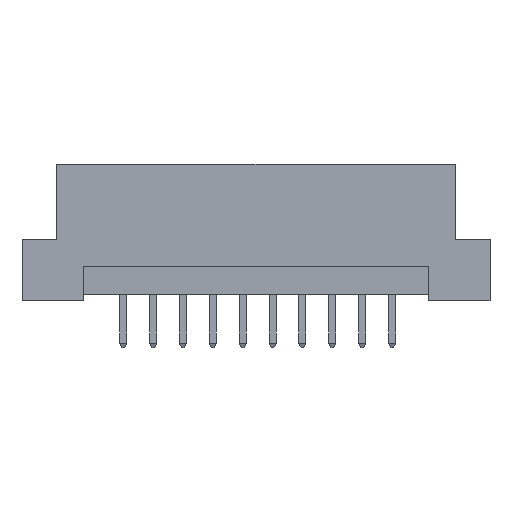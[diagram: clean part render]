
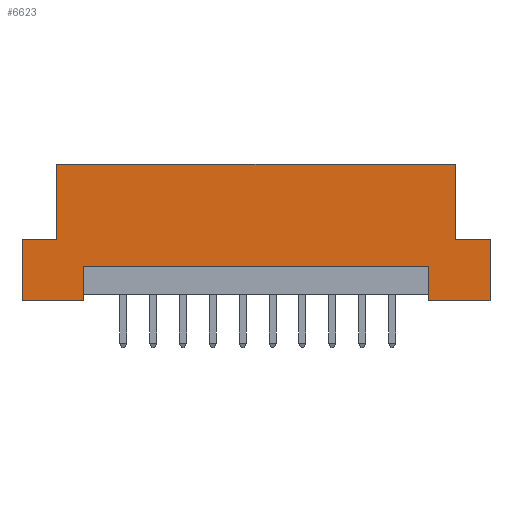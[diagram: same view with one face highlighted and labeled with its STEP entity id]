
A CAD part, front view. The second image highlights one B-rep face of the part: STEP entity #6623.
In plain terms, the highlighted planar face has unit normal (0, -1, 0).
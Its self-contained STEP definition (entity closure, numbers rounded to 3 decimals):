
#6 = EDGE_CURVE ( 'NONE', #1249, #6115, #4848, .T. ) ;
#70 = LINE ( 'NONE', #2786, #2813 ) ;
#89 = ORIENTED_EDGE ( 'NONE', *, *, #6, .F. ) ;
#136 = EDGE_CURVE ( 'NONE', #4569, #6546, #3872, .T. ) ;
#197 = CARTESIAN_POINT ( 'NONE',  ( 14.69, 0., 0. ) ) ;
#205 = EDGE_CURVE ( 'NONE', #6596, #249, #2194, .T. ) ;
#227 = LINE ( 'NONE', #7023, #6987 ) ;
#249 = VERTEX_POINT ( 'NONE', #197 ) ;
#285 = DIRECTION ( 'NONE',  ( 0., 0., 1. ) ) ;
#328 = PLANE ( 'NONE',  #820 ) ;
#412 = DIRECTION ( 'NONE',  ( 1., 0., 0. ) ) ;
#429 = CARTESIAN_POINT ( 'NONE',  ( 16.94, 0., 5.2 ) ) ;
#633 = LINE ( 'NONE', #2880, #651 ) ;
#637 = CARTESIAN_POINT ( 'NONE',  ( -19.9, 0., 0. ) ) ;
#649 = VERTEX_POINT ( 'NONE', #3262 ) ;
#651 = VECTOR ( 'NONE', #6717, 1000. ) ;
#717 = CARTESIAN_POINT ( 'NONE',  ( 16.94, 0., 5.2 ) ) ;
#820 = AXIS2_PLACEMENT_3D ( 'NONE', #3805, #5403, #285 ) ;
#832 = DIRECTION ( 'NONE',  ( 0., 0., 1. ) ) ;
#866 = CARTESIAN_POINT ( 'NONE',  ( -19.9, 0., 0. ) ) ;
#998 = VERTEX_POINT ( 'NONE', #6518 ) ;
#1003 = EDGE_CURVE ( 'NONE', #6596, #4569, #5958, .T. ) ;
#1139 = EDGE_CURVE ( 'NONE', #5702, #4006, #1870, .T. ) ;
#1249 = VERTEX_POINT ( 'NONE', #637 ) ;
#1346 = DIRECTION ( 'NONE',  ( 1., 0., 0. ) ) ;
#1409 = VECTOR ( 'NONE', #5511, 1000. ) ;
#1461 = VECTOR ( 'NONE', #832, 1000. ) ;
#1639 = ORIENTED_EDGE ( 'NONE', *, *, #205, .T. ) ;
#1870 = LINE ( 'NONE', #3524, #4926 ) ;
#2071 = VECTOR ( 'NONE', #5396, 1000. ) ;
#2151 = VERTEX_POINT ( 'NONE', #3751 ) ;
#2194 = LINE ( 'NONE', #6733, #7275 ) ;
#2226 = CARTESIAN_POINT ( 'NONE',  ( -14.69, 0., 0.5 ) ) ;
#2272 = VECTOR ( 'NONE', #3102, 1000. ) ;
#2786 = CARTESIAN_POINT ( 'NONE',  ( -16.94, 0., 5.2 ) ) ;
#2813 = VECTOR ( 'NONE', #6864, 1000. ) ;
#2865 = ORIENTED_EDGE ( 'NONE', *, *, #7058, .F. ) ;
#2880 = CARTESIAN_POINT ( 'NONE',  ( -19.9, 0., 0. ) ) ;
#2933 = ORIENTED_EDGE ( 'NONE', *, *, #136, .F. ) ;
#3102 = DIRECTION ( 'NONE',  ( -1., 0., 0. ) ) ;
#3109 = CARTESIAN_POINT ( 'NONE',  ( 14.69, 0., 2.9 ) ) ;
#3138 = EDGE_CURVE ( 'NONE', #4006, #249, #5955, .T. ) ;
#3166 = CARTESIAN_POINT ( 'NONE',  ( -19.9, 0., 11.6 ) ) ;
#3174 = VERTEX_POINT ( 'NONE', #717 ) ;
#3202 = VECTOR ( 'NONE', #412, 1000. ) ;
#3262 = CARTESIAN_POINT ( 'NONE',  ( -16.94, 0., 5.2 ) ) ;
#3363 = CARTESIAN_POINT ( 'NONE',  ( 19.9, 0., 0. ) ) ;
#3495 = ORIENTED_EDGE ( 'NONE', *, *, #4456, .F. ) ;
#3524 = CARTESIAN_POINT ( 'NONE',  ( 19.9, 0., 0. ) ) ;
#3733 = CARTESIAN_POINT ( 'NONE',  ( -14.69, 0., 2.9 ) ) ;
#3751 = CARTESIAN_POINT ( 'NONE',  ( 16.94, 0., 11.6 ) ) ;
#3805 = CARTESIAN_POINT ( 'NONE',  ( -19.9, 0., 11.6 ) ) ;
#3861 = LINE ( 'NONE', #3166, #3202 ) ;
#3872 = LINE ( 'NONE', #2226, #6681 ) ;
#4006 = VERTEX_POINT ( 'NONE', #3363 ) ;
#4076 = ORIENTED_EDGE ( 'NONE', *, *, #7041, .F. ) ;
#4236 = ORIENTED_EDGE ( 'NONE', *, *, #1003, .F. ) ;
#4257 = CARTESIAN_POINT ( 'NONE',  ( -19.9, 0., 5.2 ) ) ;
#4360 = FACE_OUTER_BOUND ( 'NONE', #5025, .T. ) ;
#4456 = EDGE_CURVE ( 'NONE', #6546, #1249, #633, .T. ) ;
#4569 = VERTEX_POINT ( 'NONE', #3733 ) ;
#4654 = DIRECTION ( 'NONE',  ( 0., 0., -1. ) ) ;
#4848 = LINE ( 'NONE', #7107, #1461 ) ;
#4870 = ORIENTED_EDGE ( 'NONE', *, *, #6548, .T. ) ;
#4926 = VECTOR ( 'NONE', #4654, 1000. ) ;
#5025 = EDGE_LOOP ( 'NONE', ( #4236, #1639, #5747, #6756, #2865, #4870, #5187, #6904, #4076, #89, #3495, #2933 ) ) ;
#5026 = DIRECTION ( 'NONE',  ( 0., 0., -1. ) ) ;
#5187 = ORIENTED_EDGE ( 'NONE', *, *, #7216, .F. ) ;
#5396 = DIRECTION ( 'NONE',  ( -1., 0., 0. ) ) ;
#5403 = DIRECTION ( 'NONE',  ( 0., 1., 0. ) ) ;
#5418 = CARTESIAN_POINT ( 'NONE',  ( 19.9, 0., 5.2 ) ) ;
#5511 = DIRECTION ( 'NONE',  ( 0., 0., 1. ) ) ;
#5558 = VECTOR ( 'NONE', #1346, 1000. ) ;
#5702 = VERTEX_POINT ( 'NONE', #5418 ) ;
#5747 = ORIENTED_EDGE ( 'NONE', *, *, #3138, .F. ) ;
#5955 = LINE ( 'NONE', #866, #2272 ) ;
#5958 = LINE ( 'NONE', #3109, #2071 ) ;
#6038 = LINE ( 'NONE', #429, #1409 ) ;
#6105 = DIRECTION ( 'NONE',  ( 0., 0., -1. ) ) ;
#6115 = VERTEX_POINT ( 'NONE', #4257 ) ;
#6269 = EDGE_CURVE ( 'NONE', #649, #998, #70, .T. ) ;
#6470 = DIRECTION ( 'NONE',  ( 1., 0., 0. ) ) ;
#6518 = CARTESIAN_POINT ( 'NONE',  ( -16.94, 0., 11.6 ) ) ;
#6546 = VERTEX_POINT ( 'NONE', #7115 ) ;
#6548 = EDGE_CURVE ( 'NONE', #3174, #2151, #6038, .T. ) ;
#6596 = VERTEX_POINT ( 'NONE', #7228 ) ;
#6623 = ADVANCED_FACE ( 'NONE', ( #4360 ), #328, .F. ) ;
#6681 = VECTOR ( 'NONE', #5026, 1000. ) ;
#6717 = DIRECTION ( 'NONE',  ( -1., 0., 0. ) ) ;
#6733 = CARTESIAN_POINT ( 'NONE',  ( 14.69, 0., 0.5 ) ) ;
#6756 = ORIENTED_EDGE ( 'NONE', *, *, #1139, .F. ) ;
#6864 = DIRECTION ( 'NONE',  ( 0., 0., 1. ) ) ;
#6904 = ORIENTED_EDGE ( 'NONE', *, *, #6269, .F. ) ;
#6987 = VECTOR ( 'NONE', #6470, 1000. ) ;
#6990 = CARTESIAN_POINT ( 'NONE',  ( -19.9, 0., 5.2 ) ) ;
#7023 = CARTESIAN_POINT ( 'NONE',  ( 19.9, 0., 5.2 ) ) ;
#7041 = EDGE_CURVE ( 'NONE', #6115, #649, #7135, .T. ) ;
#7058 = EDGE_CURVE ( 'NONE', #3174, #5702, #227, .T. ) ;
#7107 = CARTESIAN_POINT ( 'NONE',  ( -19.9, 0., 0. ) ) ;
#7115 = CARTESIAN_POINT ( 'NONE',  ( -14.69, 0., 0. ) ) ;
#7135 = LINE ( 'NONE', #6990, #5558 ) ;
#7216 = EDGE_CURVE ( 'NONE', #998, #2151, #3861, .T. ) ;
#7228 = CARTESIAN_POINT ( 'NONE',  ( 14.69, 0., 2.9 ) ) ;
#7275 = VECTOR ( 'NONE', #6105, 1000. ) ;
